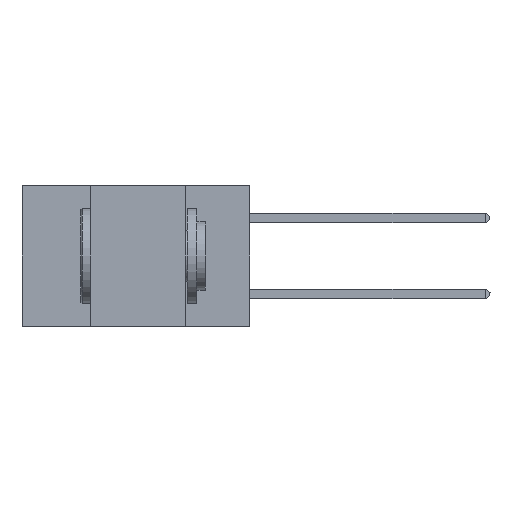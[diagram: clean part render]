
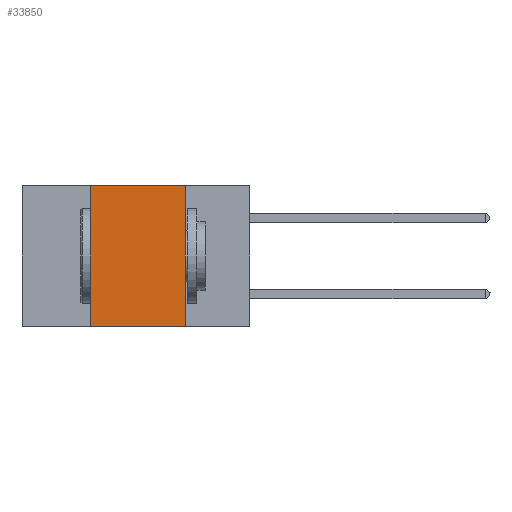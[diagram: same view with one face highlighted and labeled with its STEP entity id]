
A CAD part, left-side view. The second image highlights one B-rep face of the part: STEP entity #33850.
In plain terms, the highlighted planar face has unit normal (-1, 0, 0).
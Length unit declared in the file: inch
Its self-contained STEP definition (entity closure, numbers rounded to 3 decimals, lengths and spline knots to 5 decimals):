
#789 = CARTESIAN_POINT ( 'NONE',  ( 0., 0.42, -0.37 ) ) ;
#4017 = EDGE_LOOP ( 'NONE', ( #13294, #27544, #4595, #12529 ) ) ;
#4123 = CARTESIAN_POINT ( 'NONE',  ( 0., 0.6, 0. ) ) ;
#4581 = VERTEX_POINT ( 'NONE', #789 ) ;
#4595 = ORIENTED_EDGE ( 'NONE', *, *, #14392, .F. ) ;
#6954 = EDGE_CURVE ( 'NONE', #16293, #24801, #9673, .T. ) ;
#8083 = EDGE_CURVE ( 'NONE', #24801, #9237, #20982, .T. ) ;
#9237 = VERTEX_POINT ( 'NONE', #13735 ) ;
#9673 = LINE ( 'NONE', #4123, #18952 ) ;
#11880 = CARTESIAN_POINT ( 'NONE',  ( 0., 0.17, 0. ) ) ;
#12123 = CARTESIAN_POINT ( 'NONE',  ( 0., 0.42, 0. ) ) ;
#12141 = CARTESIAN_POINT ( 'NONE',  ( 0., 0.6, -0.37 ) ) ;
#12529 = ORIENTED_EDGE ( 'NONE', *, *, #27800, .T. ) ;
#13294 = ORIENTED_EDGE ( 'NONE', *, *, #8083, .F. ) ;
#13399 = CARTESIAN_POINT ( 'NONE',  ( 0., 0.42, 0. ) ) ;
#13735 = CARTESIAN_POINT ( 'NONE',  ( 0., 0.17, -0.37 ) ) ;
#13909 = DIRECTION ( 'NONE',  ( 0., 0., -1. ) ) ;
#14392 = EDGE_CURVE ( 'NONE', #4581, #16293, #28962, .T. ) ;
#15401 = CARTESIAN_POINT ( 'NONE',  ( 0., 0.6, 0. ) ) ;
#16293 = VERTEX_POINT ( 'NONE', #12123 ) ;
#17534 = DIRECTION ( 'NONE',  ( 0., -1., 0. ) ) ;
#18952 = VECTOR ( 'NONE', #20694, 39.37008 ) ;
#19335 = CARTESIAN_POINT ( 'NONE',  ( 0., 0.17, 0. ) ) ;
#20499 = VECTOR ( 'NONE', #31981, 39.37008 ) ;
#20694 = DIRECTION ( 'NONE',  ( 0., -1., 0. ) ) ;
#20751 = PLANE ( 'NONE',  #26906 ) ;
#20982 = LINE ( 'NONE', #19335, #29504 ) ;
#23590 = DIRECTION ( 'NONE',  ( 0., 0., -1. ) ) ;
#24801 = VERTEX_POINT ( 'NONE', #11880 ) ;
#26906 = AXIS2_PLACEMENT_3D ( 'NONE', #15401, #34350, #23590 ) ;
#27544 = ORIENTED_EDGE ( 'NONE', *, *, #6954, .F. ) ;
#27800 = EDGE_CURVE ( 'NONE', #4581, #9237, #29714, .T. ) ;
#28042 = FACE_OUTER_BOUND ( 'NONE', #4017, .T. ) ;
#28962 = LINE ( 'NONE', #13399, #20499 ) ;
#29504 = VECTOR ( 'NONE', #13909, 39.37008 ) ;
#29714 = LINE ( 'NONE', #12141, #34336 ) ;
#31981 = DIRECTION ( 'NONE',  ( 0., 0., 1. ) ) ;
#33850 = ADVANCED_FACE ( 'NONE', ( #28042 ), #20751, .F. ) ;
#34336 = VECTOR ( 'NONE', #17534, 39.37008 ) ;
#34350 = DIRECTION ( 'NONE',  ( 1., 0., 0. ) ) ;
